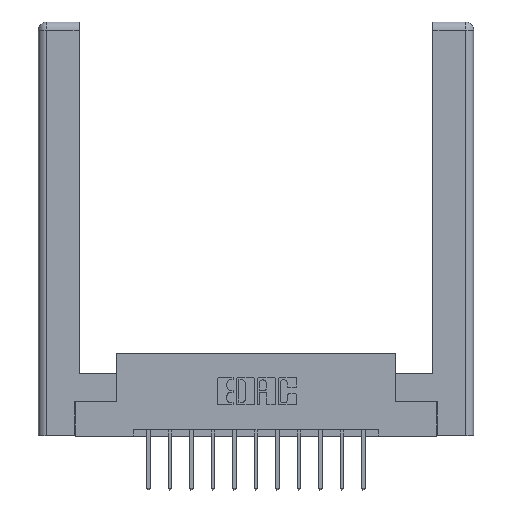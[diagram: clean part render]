
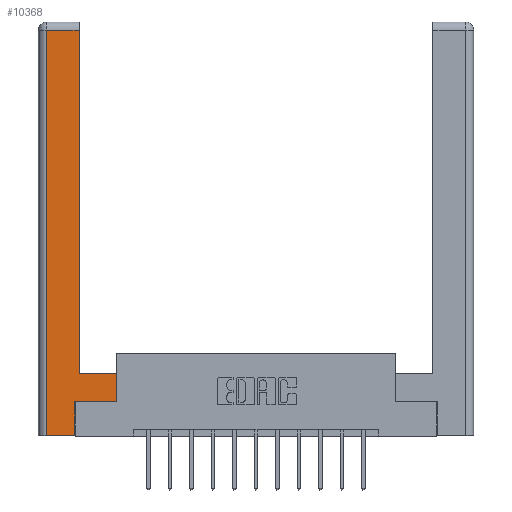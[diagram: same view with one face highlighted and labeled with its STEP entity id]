
A CAD part, top view. The second image highlights one B-rep face of the part: STEP entity #10368.
In plain terms, the highlighted planar face has unit normal (0, 0, 1).
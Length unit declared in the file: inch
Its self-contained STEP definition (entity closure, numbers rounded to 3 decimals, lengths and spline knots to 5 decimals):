
#230 = ORIENTED_EDGE ( 'NONE', *, *, #7455, .T. ) ;
#437 = DIRECTION ( 'NONE',  ( 0., 1., 0. ) ) ;
#865 = DIRECTION ( 'NONE',  ( 0., 1., 0. ) ) ;
#940 = LINE ( 'NONE', #4710, #13097 ) ;
#1413 = VERTEX_POINT ( 'NONE', #13899 ) ;
#1902 = ORIENTED_EDGE ( 'NONE', *, *, #12522, .T. ) ;
#2003 = CARTESIAN_POINT ( 'NONE',  ( 0.0615, 0., 0. ) ) ;
#2131 = DIRECTION ( 'NONE',  ( -1., 0., 0. ) ) ;
#2278 = ORIENTED_EDGE ( 'NONE', *, *, #9067, .T. ) ;
#2555 = LINE ( 'NONE', #13898, #12273 ) ;
#2855 = LINE ( 'NONE', #12672, #8727 ) ;
#3266 = VECTOR ( 'NONE', #10793, 39.37008 ) ;
#3271 = LINE ( 'NONE', #11773, #12267 ) ;
#3446 = LINE ( 'NONE', #11975, #3266 ) ;
#3824 = CARTESIAN_POINT ( 'NONE',  ( 0.0615, 2.94, 0. ) ) ;
#3875 = DIRECTION ( 'NONE',  ( 1., 0., 0. ) ) ;
#4586 = LINE ( 'NONE', #6635, #7707 ) ;
#4710 = CARTESIAN_POINT ( 'NONE',  ( 0.265, 0., 0. ) ) ;
#5231 = CARTESIAN_POINT ( 'NONE',  ( 0.565, 0.245, 0. ) ) ;
#5530 = PLANE ( 'NONE',  #10366 ) ;
#5596 = EDGE_CURVE ( 'NONE', #14815, #11104, #3446, .T. ) ;
#5857 = CARTESIAN_POINT ( 'NONE',  ( 0.265, 0., 0. ) ) ;
#5926 = ORIENTED_EDGE ( 'NONE', *, *, #5596, .T. ) ;
#6233 = LINE ( 'NONE', #9231, #13063 ) ;
#6591 = FACE_OUTER_BOUND ( 'NONE', #7400, .T. ) ;
#6635 = CARTESIAN_POINT ( 'NONE',  ( 0.295, 3., 0. ) ) ;
#6653 = CARTESIAN_POINT ( 'NONE',  ( 0., 0., 0. ) ) ;
#7129 = LINE ( 'NONE', #13401, #9714 ) ;
#7143 = CARTESIAN_POINT ( 'NONE',  ( 0.295, 2.94, 0. ) ) ;
#7400 = EDGE_LOOP ( 'NONE', ( #11661, #5926, #13677, #230, #2278, #12354, #1902, #11166 ) ) ;
#7455 = EDGE_CURVE ( 'NONE', #7690, #8225, #940, .T. ) ;
#7690 = VERTEX_POINT ( 'NONE', #2003 ) ;
#7707 = VECTOR ( 'NONE', #11307, 39.37008 ) ;
#7989 = DIRECTION ( 'NONE',  ( 1., 0., 0. ) ) ;
#8225 = VERTEX_POINT ( 'NONE', #5857 ) ;
#8727 = VECTOR ( 'NONE', #865, 39.37008 ) ;
#9067 = EDGE_CURVE ( 'NONE', #8225, #14216, #7129, .T. ) ;
#9080 = DIRECTION ( 'NONE',  ( 0., -1., 0. ) ) ;
#9231 = CARTESIAN_POINT ( 'NONE',  ( 0.0615, 0., 0. ) ) ;
#9339 = EDGE_CURVE ( 'NONE', #14216, #15049, #3271, .T. ) ;
#9714 = VECTOR ( 'NONE', #437, 39.37008 ) ;
#10320 = EDGE_CURVE ( 'NONE', #11104, #7690, #6233, .T. ) ;
#10346 = DIRECTION ( 'NONE',  ( -1., 0., 0. ) ) ;
#10366 = AXIS2_PLACEMENT_3D ( 'NONE', #6653, #12616, #2131 ) ;
#10368 = ADVANCED_FACE ( 'NONE', ( #6591 ), #5530, .F. ) ;
#10465 = VERTEX_POINT ( 'NONE', #11630 ) ;
#10793 = DIRECTION ( 'NONE',  ( -1., 0., 0. ) ) ;
#10842 = EDGE_CURVE ( 'NONE', #1413, #10465, #2555, .T. ) ;
#11104 = VERTEX_POINT ( 'NONE', #3824 ) ;
#11166 = ORIENTED_EDGE ( 'NONE', *, *, #10842, .T. ) ;
#11307 = DIRECTION ( 'NONE',  ( 0., 1., 0. ) ) ;
#11630 = CARTESIAN_POINT ( 'NONE',  ( 0.295, 0.45, 0. ) ) ;
#11661 = ORIENTED_EDGE ( 'NONE', *, *, #14513, .T. ) ;
#11773 = CARTESIAN_POINT ( 'NONE',  ( 0.565, 0.245, 0. ) ) ;
#11975 = CARTESIAN_POINT ( 'NONE',  ( 0.0615, 2.94, 0. ) ) ;
#12267 = VECTOR ( 'NONE', #3875, 39.37008 ) ;
#12273 = VECTOR ( 'NONE', #10346, 39.37008 ) ;
#12354 = ORIENTED_EDGE ( 'NONE', *, *, #9339, .T. ) ;
#12522 = EDGE_CURVE ( 'NONE', #15049, #1413, #2855, .T. ) ;
#12616 = DIRECTION ( 'NONE',  ( 0., 0., -1. ) ) ;
#12672 = CARTESIAN_POINT ( 'NONE',  ( 0.565, 0.45, 0. ) ) ;
#13063 = VECTOR ( 'NONE', #9080, 39.37008 ) ;
#13097 = VECTOR ( 'NONE', #7989, 39.37008 ) ;
#13401 = CARTESIAN_POINT ( 'NONE',  ( 0.265, 0.245, 0. ) ) ;
#13677 = ORIENTED_EDGE ( 'NONE', *, *, #10320, .T. ) ;
#13898 = CARTESIAN_POINT ( 'NONE',  ( 0.295, 0.45, 0. ) ) ;
#13899 = CARTESIAN_POINT ( 'NONE',  ( 0.565, 0.45, 0. ) ) ;
#14152 = CARTESIAN_POINT ( 'NONE',  ( 0.265, 0.245, 0. ) ) ;
#14216 = VERTEX_POINT ( 'NONE', #14152 ) ;
#14513 = EDGE_CURVE ( 'NONE', #10465, #14815, #4586, .T. ) ;
#14815 = VERTEX_POINT ( 'NONE', #7143 ) ;
#15049 = VERTEX_POINT ( 'NONE', #5231 ) ;
